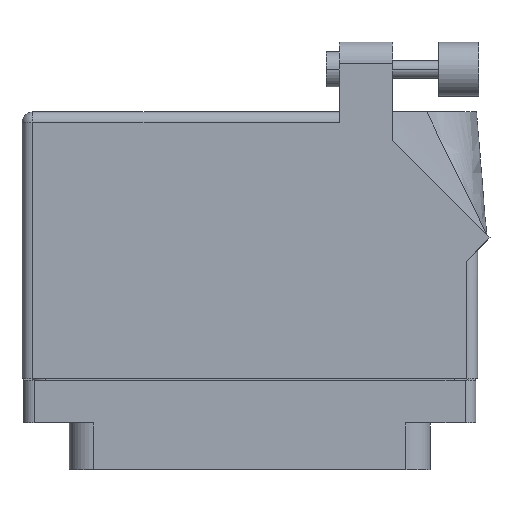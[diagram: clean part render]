
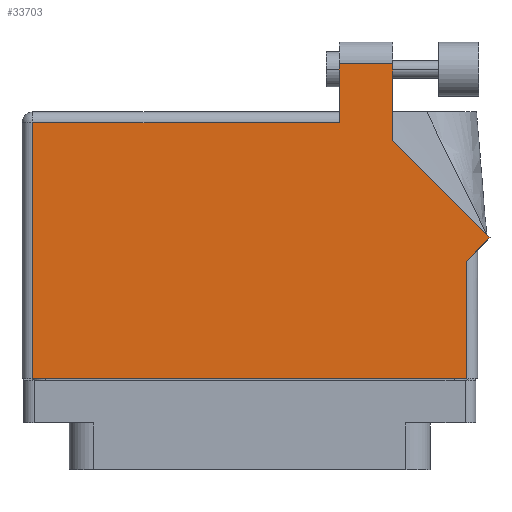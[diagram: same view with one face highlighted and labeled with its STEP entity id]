
A CAD part, front view. The second image highlights one B-rep face of the part: STEP entity #33703.
In plain terms, the highlighted face is planar.
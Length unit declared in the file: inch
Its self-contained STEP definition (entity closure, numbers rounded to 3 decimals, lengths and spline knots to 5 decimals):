
#9 = CARTESIAN_POINT ( 'NONE',  ( 0.513, 1.705, 0.455 ) ) ;
#1316 = VECTOR ( 'NONE', #51742, 39.37008 ) ;
#1318 = VECTOR ( 'NONE', #10043, 39.37008 ) ;
#2114 = VECTOR ( 'NONE', #46852, 39.37008 ) ;
#2822 = VERTEX_POINT ( 'NONE', #51017 ) ;
#2826 = ORIENTED_EDGE ( 'NONE', *, *, #22868, .T. ) ;
#3632 = EDGE_CURVE ( 'NONE', #4898, #15242, #44855, .T. ) ;
#4898 = VERTEX_POINT ( 'NONE', #33804 ) ;
#6184 = CARTESIAN_POINT ( 'NONE',  ( 1.244, -0.1, 0.455 ) ) ;
#6268 = ORIENTED_EDGE ( 'NONE', *, *, #3632, .T. ) ;
#6358 = EDGE_CURVE ( 'NONE', #26319, #34879, #50234, .T. ) ;
#7120 = LINE ( 'NONE', #46685, #2114 ) ;
#9103 = VERTEX_POINT ( 'NONE', #10176 ) ;
#10043 = DIRECTION ( 'NONE',  ( 0., 1., 0. ) ) ;
#10176 = CARTESIAN_POINT ( 'NONE',  ( -1.244, -0.1, 0.455 ) ) ;
#11194 = LINE ( 'NONE', #45142, #32598 ) ;
#11463 = CARTESIAN_POINT ( 'NONE',  ( 0.513, 1.43, 0.455 ) ) ;
#12510 = CARTESIAN_POINT ( 'NONE',  ( 1.37671, 0.70771, 0.455 ) ) ;
#12787 = CARTESIAN_POINT ( 'NONE',  ( -1.306, 1.368, 0.455 ) ) ;
#13128 = VERTEX_POINT ( 'NONE', #12510 ) ;
#14441 = EDGE_CURVE ( 'NONE', #13128, #38773, #27945, .T. ) ;
#14688 = DIRECTION ( 'NONE',  ( -1., 0., 0. ) ) ;
#15242 = VERTEX_POINT ( 'NONE', #9 ) ;
#16344 = EDGE_CURVE ( 'NONE', #15242, #2822, #34596, .T. ) ;
#18532 = EDGE_CURVE ( 'NONE', #2822, #45300, #44151, .T. ) ;
#18860 = EDGE_CURVE ( 'NONE', #45300, #9103, #7120, .T. ) ;
#20100 = CARTESIAN_POINT ( 'NONE',  ( -1.306, 1.43, 0.455 ) ) ;
#20312 = LINE ( 'NONE', #43904, #50991 ) ;
#20728 = VECTOR ( 'NONE', #48542, 39.37008 ) ;
#20885 = ORIENTED_EDGE ( 'NONE', *, *, #6358, .T. ) ;
#20941 = ORIENTED_EDGE ( 'NONE', *, *, #14441, .T. ) ;
#22373 = CARTESIAN_POINT ( 'NONE',  ( 0.82, 1.26442, 0.455 ) ) ;
#22813 = VECTOR ( 'NONE', #28174, 39.37008 ) ;
#22868 = EDGE_CURVE ( 'NONE', #9103, #26319, #20312, .T. ) ;
#23532 = EDGE_LOOP ( 'NONE', ( #28823, #6268, #42237, #38858, #29085, #2826, #20885, #44643, #20941 ) ) ;
#26319 = VERTEX_POINT ( 'NONE', #6184 ) ;
#27214 = FACE_OUTER_BOUND ( 'NONE', #23532, .T. ) ;
#27945 = LINE ( 'NONE', #34692, #48008 ) ;
#28174 = DIRECTION ( 'NONE',  ( -1., 0., 0. ) ) ;
#28823 = ORIENTED_EDGE ( 'NONE', *, *, #31422, .T. ) ;
#29085 = ORIENTED_EDGE ( 'NONE', *, *, #18860, .T. ) ;
#31422 = EDGE_CURVE ( 'NONE', #38773, #4898, #47645, .T. ) ;
#32392 = DIRECTION ( 'NONE',  ( -1., 0., 0. ) ) ;
#32598 = VECTOR ( 'NONE', #32602, 39.37008 ) ;
#32602 = DIRECTION ( 'NONE',  ( 0.707, 0.707, 0. ) ) ;
#33703 = ADVANCED_FACE ( 'NONE', ( #27214 ), #51276, .F. ) ;
#33804 = CARTESIAN_POINT ( 'NONE',  ( 0.82, 1.705, 0.455 ) ) ;
#33985 = DIRECTION ( 'NONE',  ( 0., 0., -1. ) ) ;
#34288 = CARTESIAN_POINT ( 'NONE',  ( 1.244, 0.637, 0.455 ) ) ;
#34596 = LINE ( 'NONE', #11463, #1316 ) ;
#34692 = CARTESIAN_POINT ( 'NONE',  ( 1.37671, 0.70771, 0.455 ) ) ;
#34879 = VERTEX_POINT ( 'NONE', #35026 ) ;
#35026 = CARTESIAN_POINT ( 'NONE',  ( 1.244, 0.575, 0.455 ) ) ;
#36265 = DIRECTION ( 'NONE',  ( 1., 0., 0. ) ) ;
#37390 = VECTOR ( 'NONE', #14688, 39.37008 ) ;
#38773 = VERTEX_POINT ( 'NONE', #22373 ) ;
#38858 = ORIENTED_EDGE ( 'NONE', *, *, #18532, .T. ) ;
#39874 = CARTESIAN_POINT ( 'NONE',  ( 0.82, 1.26442, 0.455 ) ) ;
#42237 = ORIENTED_EDGE ( 'NONE', *, *, #16344, .T. ) ;
#42519 = EDGE_CURVE ( 'NONE', #34879, #13128, #11194, .T. ) ;
#42738 = DIRECTION ( 'NONE',  ( -0.707, 0.707, 0. ) ) ;
#43854 = CARTESIAN_POINT ( 'NONE',  ( -1.244, 1.368, 0.455 ) ) ;
#43904 = CARTESIAN_POINT ( 'NONE',  ( -1.306, -0.1, 0.455 ) ) ;
#44151 = LINE ( 'NONE', #12787, #22813 ) ;
#44643 = ORIENTED_EDGE ( 'NONE', *, *, #42519, .T. ) ;
#44855 = LINE ( 'NONE', #46896, #37390 ) ;
#45142 = CARTESIAN_POINT ( 'NONE',  ( 1.306, 0.637, 0.455 ) ) ;
#45300 = VERTEX_POINT ( 'NONE', #43854 ) ;
#46685 = CARTESIAN_POINT ( 'NONE',  ( -1.244, -0.1, 0.455 ) ) ;
#46852 = DIRECTION ( 'NONE',  ( 0., -1., 0. ) ) ;
#46896 = CARTESIAN_POINT ( 'NONE',  ( 0.513, 1.705, 0.455 ) ) ;
#47645 = LINE ( 'NONE', #39874, #20728 ) ;
#48008 = VECTOR ( 'NONE', #42738, 39.37008 ) ;
#48542 = DIRECTION ( 'NONE',  ( 0., 1., 0. ) ) ;
#48825 = AXIS2_PLACEMENT_3D ( 'NONE', #20100, #33985, #32392 ) ;
#50234 = LINE ( 'NONE', #34288, #1318 ) ;
#50991 = VECTOR ( 'NONE', #36265, 39.37008 ) ;
#51017 = CARTESIAN_POINT ( 'NONE',  ( 0.513, 1.368, 0.455 ) ) ;
#51276 = PLANE ( 'NONE',  #48825 ) ;
#51742 = DIRECTION ( 'NONE',  ( 0., -1., 0. ) ) ;
